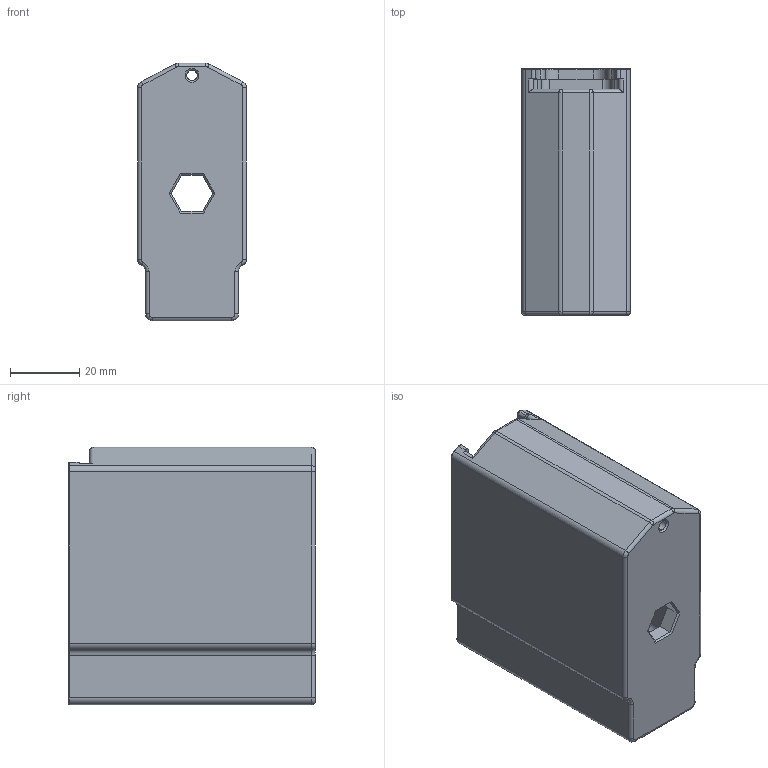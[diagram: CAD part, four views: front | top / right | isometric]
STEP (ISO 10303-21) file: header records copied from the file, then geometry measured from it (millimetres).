
FILE_DESCRIPTION(/* description */ (''),/* implementation_level */ '2;1');
FILE_NAME(/* name */ '41f20733-90c5-4bc1-81e3-1afe90c4ad54.stp',/* time_stamp */ '2019-04-30T20:32:40-04:00',/* author */ ('suzuki450ltr'),/* organization */ (''),/* preprocessor_version */ 'ST-DEVELOPER v18',/* originating_system */ 'Autodesk Translation Framework v8.2.0.1029',/* authorisation */ '');
FILE_SCHEMA (('AUTOMOTIVE_DESIGN { 1 0 10303 214 3 1 1 }'));
Length unit declared in the file: millimetre
Products named in the file (1): Hex Mag Extension
Bounding box: 31.35 x 71 x 74.15 mm (x, y, z)
Volume: 79103.3 mm3; surface area: 29170.7 mm2
Topology: 1 solids, 1 shells, 197 faces, 466 edges, 269 vertices
Faces by surface type: cylinder 86, plane 53, torus 36, bspline 14, sphere 6, cone 2
Full cylindrical faces by diameter (mm): 3 x1
Entity records: 5774 total; most frequent: CARTESIAN_POINT 1123, DIRECTION 1059, ORIENTED_EDGE 928, EDGE_CURVE 464, AXIS2_PLACEMENT_3D 415, VERTEX_POINT 269, LINE 229, VECTOR 229
